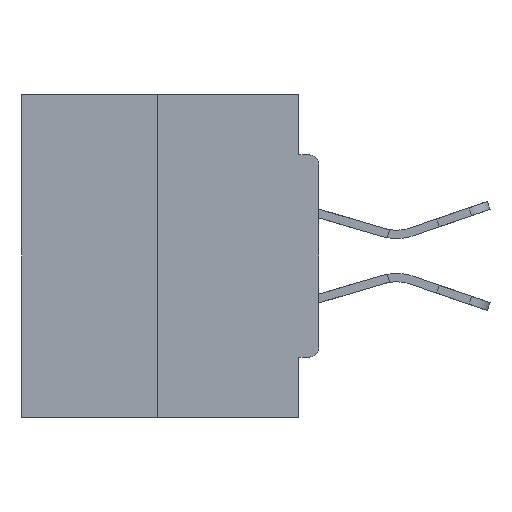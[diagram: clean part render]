
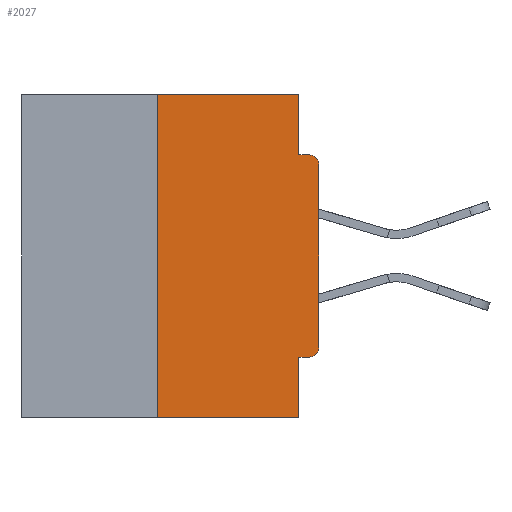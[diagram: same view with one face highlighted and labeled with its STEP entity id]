
A CAD part, left-side view. The second image highlights one B-rep face of the part: STEP entity #2027.
In plain terms, the highlighted planar face has unit normal (-1, 0, 0).
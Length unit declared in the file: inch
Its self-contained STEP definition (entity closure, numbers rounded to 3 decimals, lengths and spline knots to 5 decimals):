
#609 = EDGE_CURVE ( 'NONE', #35467, #24430, #13079, .T. ) ;
#1152 = ORIENTED_EDGE ( 'NONE', *, *, #21885, .F. ) ;
#1234 = VECTOR ( 'NONE', #28092, 39.37008 ) ;
#1707 = VERTEX_POINT ( 'NONE', #21052 ) ;
#2027 = ADVANCED_FACE ( 'NONE', ( #35571 ), #27704, .F. ) ;
#2352 = DIRECTION ( 'NONE',  ( 0., 0., -1. ) ) ;
#3588 = EDGE_LOOP ( 'NONE', ( #4556, #1152, #16498, #36088, #39237, #9486, #19513, #11018, #27614, #19995 ) ) ;
#4556 = ORIENTED_EDGE ( 'NONE', *, *, #12522, .F. ) ;
#5981 = EDGE_CURVE ( 'NONE', #32161, #10005, #30279, .T. ) ;
#6322 = CARTESIAN_POINT ( 'NONE',  ( 0., 0., 0. ) ) ;
#6627 = DIRECTION ( 'NONE',  ( 0., 0., -1. ) ) ;
#7139 = CARTESIAN_POINT ( 'NONE',  ( 0., 0., -0.4065 ) ) ;
#7312 = LINE ( 'NONE', #24966, #24512 ) ;
#8263 = AXIS2_PLACEMENT_3D ( 'NONE', #37239, #17960, #2352 ) ;
#9486 = ORIENTED_EDGE ( 'NONE', *, *, #36377, .T. ) ;
#9846 = CARTESIAN_POINT ( 'NONE',  ( 0., 0.015, -0.4065 ) ) ;
#9937 = CARTESIAN_POINT ( 'NONE',  ( 0., 0., -0.1085 ) ) ;
#10005 = VERTEX_POINT ( 'NONE', #34293 ) ;
#10068 = CARTESIAN_POINT ( 'NONE',  ( 0., 0.25, 0. ) ) ;
#10309 = CARTESIAN_POINT ( 'NONE',  ( 0., 0.25, 0. ) ) ;
#10326 = CARTESIAN_POINT ( 'NONE',  ( 0., 0., -0.3915 ) ) ;
#11018 = ORIENTED_EDGE ( 'NONE', *, *, #30174, .T. ) ;
#11269 = VECTOR ( 'NONE', #31999, 39.37008 ) ;
#11619 = VECTOR ( 'NONE', #32302, 39.37008 ) ;
#11804 = CARTESIAN_POINT ( 'NONE',  ( 0., 0.46, -0.5 ) ) ;
#12181 = CARTESIAN_POINT ( 'NONE',  ( 0., 0.031, 0. ) ) ;
#12522 = EDGE_CURVE ( 'NONE', #37541, #18003, #23303, .T. ) ;
#12689 = CARTESIAN_POINT ( 'NONE',  ( 0., 0.25, -0.5 ) ) ;
#13079 = LINE ( 'NONE', #6322, #35691 ) ;
#13362 = VECTOR ( 'NONE', #6627, 39.37008 ) ;
#14480 = LINE ( 'NONE', #11804, #34638 ) ;
#14635 = CIRCLE ( 'NONE', #22076, 0.015 ) ;
#16498 = ORIENTED_EDGE ( 'NONE', *, *, #30328, .T. ) ;
#17960 = DIRECTION ( 'NONE',  ( 1., 0., 0. ) ) ;
#18003 = VERTEX_POINT ( 'NONE', #12181 ) ;
#19513 = ORIENTED_EDGE ( 'NONE', *, *, #609, .T. ) ;
#19995 = ORIENTED_EDGE ( 'NONE', *, *, #33972, .F. ) ;
#20540 = DIRECTION ( 'NONE',  ( -1., 0., 0. ) ) ;
#21052 = CARTESIAN_POINT ( 'NONE',  ( 0., 0.031, -0.4065 ) ) ;
#21121 = AXIS2_PLACEMENT_3D ( 'NONE', #32029, #22669, #25968 ) ;
#21563 = VERTEX_POINT ( 'NONE', #36775 ) ;
#21885 = EDGE_CURVE ( 'NONE', #23736, #37541, #39786, .T. ) ;
#22076 = AXIS2_PLACEMENT_3D ( 'NONE', #27386, #20540, #27254 ) ;
#22174 = LINE ( 'NONE', #28187, #13362 ) ;
#22410 = LINE ( 'NONE', #7139, #11619 ) ;
#22669 = DIRECTION ( 'NONE',  ( -1., 0., 0. ) ) ;
#23303 = LINE ( 'NONE', #40108, #1234 ) ;
#23736 = VERTEX_POINT ( 'NONE', #12689 ) ;
#24430 = VERTEX_POINT ( 'NONE', #9937 ) ;
#24512 = VECTOR ( 'NONE', #32101, 39.37008 ) ;
#24966 = CARTESIAN_POINT ( 'NONE',  ( 0., 0.031, -0.5 ) ) ;
#25256 = DIRECTION ( 'NONE',  ( 0., 0., 1. ) ) ;
#25968 = DIRECTION ( 'NONE',  ( 0., 0., -1. ) ) ;
#27254 = DIRECTION ( 'NONE',  ( 0., 0., -1. ) ) ;
#27386 = CARTESIAN_POINT ( 'NONE',  ( 0., 0.015, -0.3915 ) ) ;
#27540 = EDGE_CURVE ( 'NONE', #1707, #21563, #7312, .T. ) ;
#27614 = ORIENTED_EDGE ( 'NONE', *, *, #5981, .F. ) ;
#27704 = PLANE ( 'NONE',  #8263 ) ;
#28092 = DIRECTION ( 'NONE',  ( 0., -1., 0. ) ) ;
#28187 = CARTESIAN_POINT ( 'NONE',  ( 0., 0.031, 0. ) ) ;
#28580 = CARTESIAN_POINT ( 'NONE',  ( 0., 0.031, -0.0935 ) ) ;
#29222 = CARTESIAN_POINT ( 'NONE',  ( 0., 0., -0.0935 ) ) ;
#30174 = EDGE_CURVE ( 'NONE', #24430, #10005, #30641, .T. ) ;
#30279 = LINE ( 'NONE', #29222, #38212 ) ;
#30328 = EDGE_CURVE ( 'NONE', #23736, #21563, #14480, .T. ) ;
#30641 = CIRCLE ( 'NONE', #21121, 0.015 ) ;
#31999 = DIRECTION ( 'NONE',  ( 0., 0., 1. ) ) ;
#32029 = CARTESIAN_POINT ( 'NONE',  ( 0., 0.015, -0.1085 ) ) ;
#32101 = DIRECTION ( 'NONE',  ( 0., 0., -1. ) ) ;
#32161 = VERTEX_POINT ( 'NONE', #28580 ) ;
#32302 = DIRECTION ( 'NONE',  ( 0., 1., 0. ) ) ;
#33972 = EDGE_CURVE ( 'NONE', #18003, #32161, #22174, .T. ) ;
#34049 = DIRECTION ( 'NONE',  ( 0., -1., 0. ) ) ;
#34293 = CARTESIAN_POINT ( 'NONE',  ( 0., 0.015, -0.0935 ) ) ;
#34638 = VECTOR ( 'NONE', #34049, 39.37008 ) ;
#35183 = DIRECTION ( 'NONE',  ( 0., -1., 0. ) ) ;
#35467 = VERTEX_POINT ( 'NONE', #10326 ) ;
#35571 = FACE_OUTER_BOUND ( 'NONE', #3588, .T. ) ;
#35691 = VECTOR ( 'NONE', #25256, 39.37008 ) ;
#36088 = ORIENTED_EDGE ( 'NONE', *, *, #27540, .F. ) ;
#36377 = EDGE_CURVE ( 'NONE', #38902, #35467, #14635, .T. ) ;
#36775 = CARTESIAN_POINT ( 'NONE',  ( 0., 0.031, -0.5 ) ) ;
#36986 = EDGE_CURVE ( 'NONE', #38902, #1707, #22410, .T. ) ;
#37239 = CARTESIAN_POINT ( 'NONE',  ( 0., 0.46, 0. ) ) ;
#37541 = VERTEX_POINT ( 'NONE', #10309 ) ;
#38212 = VECTOR ( 'NONE', #35183, 39.37008 ) ;
#38902 = VERTEX_POINT ( 'NONE', #9846 ) ;
#39237 = ORIENTED_EDGE ( 'NONE', *, *, #36986, .F. ) ;
#39786 = LINE ( 'NONE', #10068, #11269 ) ;
#40108 = CARTESIAN_POINT ( 'NONE',  ( 0., 0.46, 0. ) ) ;
